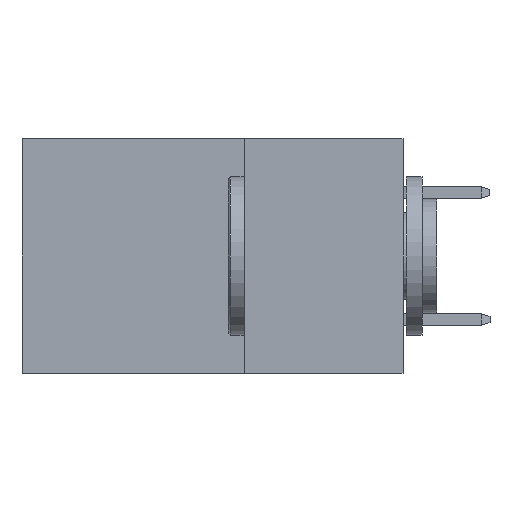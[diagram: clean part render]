
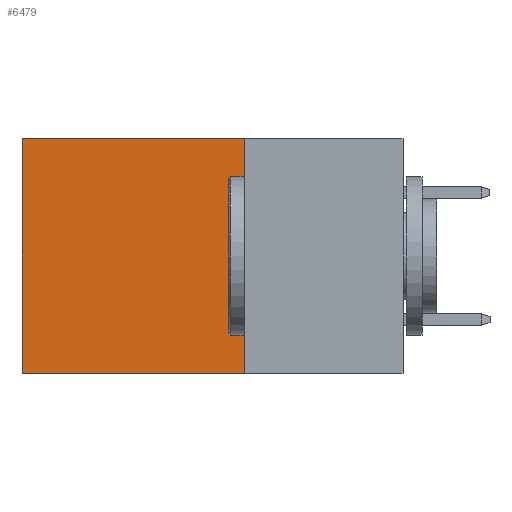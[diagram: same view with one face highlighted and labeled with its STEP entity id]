
A CAD part, left-side view. The second image highlights one B-rep face of the part: STEP entity #6479.
In plain terms, the highlighted planar face has unit normal (-1, 0, 0).
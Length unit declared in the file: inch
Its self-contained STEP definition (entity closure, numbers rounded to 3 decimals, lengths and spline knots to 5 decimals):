
#152 = VECTOR ( 'NONE', #2880, 39.37008 ) ;
#203 = LINE ( 'NONE', #8672, #152 ) ;
#491 = DIRECTION ( 'NONE',  ( 0., 0., -1. ) ) ;
#565 = FACE_OUTER_BOUND ( 'NONE', #10038, .T. ) ;
#674 = AXIS2_PLACEMENT_3D ( 'NONE', #10726, #6595, #9940 ) ;
#1094 = VECTOR ( 'NONE', #491, 39.37008 ) ;
#1315 = LINE ( 'NONE', #6965, #1094 ) ;
#1505 = VERTEX_POINT ( 'NONE', #10614 ) ;
#1699 = ORIENTED_EDGE ( 'NONE', *, *, #5010, .T. ) ;
#2563 = EDGE_CURVE ( 'NONE', #1505, #8740, #10191, .T. ) ;
#2611 = CARTESIAN_POINT ( 'NONE',  ( 0.2875, 0.25, -0.37 ) ) ;
#2627 = EDGE_CURVE ( 'NONE', #9774, #3029, #8079, .T. ) ;
#2775 = ORIENTED_EDGE ( 'NONE', *, *, #2627, .T. ) ;
#2880 = DIRECTION ( 'NONE',  ( 0., 0., -1. ) ) ;
#3029 = VERTEX_POINT ( 'NONE', #5657 ) ;
#3628 = VECTOR ( 'NONE', #4336, 39.37008 ) ;
#4336 = DIRECTION ( 'NONE',  ( 0., 1., 0. ) ) ;
#5010 = EDGE_CURVE ( 'NONE', #3029, #8740, #1315, .T. ) ;
#5243 = ORIENTED_EDGE ( 'NONE', *, *, #2563, .F. ) ;
#5488 = DIRECTION ( 'NONE',  ( 0., 1., 0. ) ) ;
#5657 = CARTESIAN_POINT ( 'NONE',  ( 0.2875, 0.6, 0. ) ) ;
#6479 = ADVANCED_FACE ( 'NONE', ( #565 ), #7364, .F. ) ;
#6484 = VECTOR ( 'NONE', #5488, 39.37008 ) ;
#6595 = DIRECTION ( 'NONE',  ( 1., 0., 0. ) ) ;
#6965 = CARTESIAN_POINT ( 'NONE',  ( 0.2875, 0.6, 0. ) ) ;
#7364 = PLANE ( 'NONE',  #674 ) ;
#7449 = ORIENTED_EDGE ( 'NONE', *, *, #10274, .F. ) ;
#8079 = LINE ( 'NONE', #10414, #6484 ) ;
#8672 = CARTESIAN_POINT ( 'NONE',  ( 0.2875, 0.25, 0. ) ) ;
#8740 = VERTEX_POINT ( 'NONE', #10759 ) ;
#9119 = CARTESIAN_POINT ( 'NONE',  ( 0.2875, 0.25, 0. ) ) ;
#9774 = VERTEX_POINT ( 'NONE', #9119 ) ;
#9940 = DIRECTION ( 'NONE',  ( 0., 0., -1. ) ) ;
#10038 = EDGE_LOOP ( 'NONE', ( #1699, #5243, #7449, #2775 ) ) ;
#10191 = LINE ( 'NONE', #2611, #3628 ) ;
#10274 = EDGE_CURVE ( 'NONE', #9774, #1505, #203, .T. ) ;
#10414 = CARTESIAN_POINT ( 'NONE',  ( 0.2875, 0.25, 0. ) ) ;
#10614 = CARTESIAN_POINT ( 'NONE',  ( 0.2875, 0.25, -0.37 ) ) ;
#10726 = CARTESIAN_POINT ( 'NONE',  ( 0.2875, 0.25, 0. ) ) ;
#10759 = CARTESIAN_POINT ( 'NONE',  ( 0.2875, 0.6, -0.37 ) ) ;
